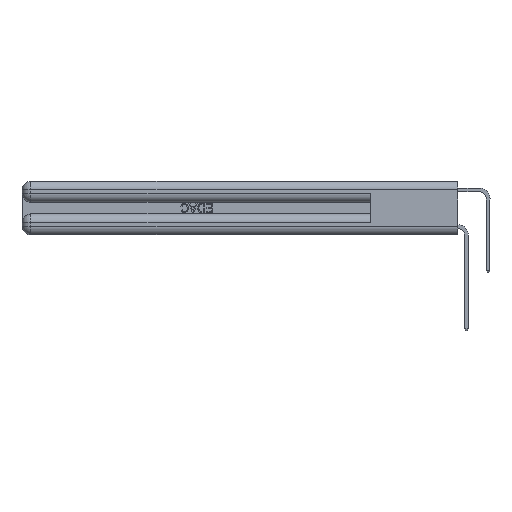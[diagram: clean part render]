
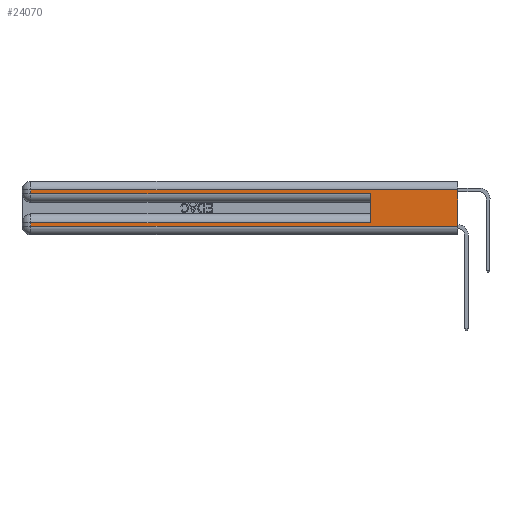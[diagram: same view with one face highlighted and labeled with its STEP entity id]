
A CAD part, left-side view. The second image highlights one B-rep face of the part: STEP entity #24070.
In plain terms, the highlighted planar face has unit normal (-1, 0, 0).
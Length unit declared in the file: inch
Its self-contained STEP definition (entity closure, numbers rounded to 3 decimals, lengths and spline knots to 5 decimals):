
#98 = EDGE_CURVE ( 'NONE', #16493, #9018, #6437, .T. ) ;
#126 = LINE ( 'NONE', #4403, #23424 ) ;
#523 = DIRECTION ( 'NONE',  ( 1., 0., 0. ) ) ;
#830 = VERTEX_POINT ( 'NONE', #20892 ) ;
#1413 = ORIENTED_EDGE ( 'NONE', *, *, #6226, .F. ) ;
#1420 = ORIENTED_EDGE ( 'NONE', *, *, #8567, .T. ) ;
#2170 = DIRECTION ( 'NONE',  ( 0., 0., -1. ) ) ;
#2882 = VERTEX_POINT ( 'NONE', #21152 ) ;
#3318 = CARTESIAN_POINT ( 'NONE',  ( 0., 0.6, 0.145 ) ) ;
#4073 = EDGE_CURVE ( 'NONE', #7418, #14097, #7111, .T. ) ;
#4253 = DIRECTION ( 'NONE',  ( 0., -1., 0. ) ) ;
#4347 = VECTOR ( 'NONE', #24216, 39.37008 ) ;
#4403 = CARTESIAN_POINT ( 'NONE',  ( 0., 0., 0.285 ) ) ;
#4581 = LINE ( 'NONE', #11133, #14206 ) ;
#4806 = CARTESIAN_POINT ( 'NONE',  ( 0., 0., 0.37 ) ) ;
#5591 = CARTESIAN_POINT ( 'NONE',  ( 0., 0., 0.31 ) ) ;
#5800 = CARTESIAN_POINT ( 'NONE',  ( 0., 2.94, 0.285 ) ) ;
#6103 = LINE ( 'NONE', #23733, #9230 ) ;
#6226 = EDGE_CURVE ( 'NONE', #2882, #830, #10009, .T. ) ;
#6437 = LINE ( 'NONE', #17681, #4347 ) ;
#6448 = EDGE_CURVE ( 'NONE', #18080, #24206, #4581, .T. ) ;
#6486 = EDGE_CURVE ( 'NONE', #2882, #16493, #17560, .T. ) ;
#6736 = CARTESIAN_POINT ( 'NONE',  ( 0., 0., 0.085 ) ) ;
#6940 = PLANE ( 'NONE',  #16130 ) ;
#7111 = LINE ( 'NONE', #9104, #25016 ) ;
#7418 = VERTEX_POINT ( 'NONE', #24120 ) ;
#8567 = EDGE_CURVE ( 'NONE', #9018, #14097, #6103, .T. ) ;
#8876 = CARTESIAN_POINT ( 'NONE',  ( 0., 2.94, 0.06 ) ) ;
#9018 = VERTEX_POINT ( 'NONE', #8876 ) ;
#9104 = CARTESIAN_POINT ( 'NONE',  ( 0., 0., 0.37 ) ) ;
#9214 = DIRECTION ( 'NONE',  ( 0., 0., -1. ) ) ;
#9230 = VECTOR ( 'NONE', #14782, 39.37008 ) ;
#9237 = ORIENTED_EDGE ( 'NONE', *, *, #98, .T. ) ;
#10009 = LINE ( 'NONE', #3318, #11490 ) ;
#10318 = VECTOR ( 'NONE', #18123, 39.37008 ) ;
#10510 = EDGE_CURVE ( 'NONE', #7418, #18080, #18402, .T. ) ;
#11133 = CARTESIAN_POINT ( 'NONE',  ( 0., 2.94, 0.37 ) ) ;
#11253 = EDGE_CURVE ( 'NONE', #24206, #830, #126, .T. ) ;
#11490 = VECTOR ( 'NONE', #27639, 39.37008 ) ;
#11905 = FACE_OUTER_BOUND ( 'NONE', #18092, .T. ) ;
#14062 = CARTESIAN_POINT ( 'NONE',  ( 0., 2.94, 0.085 ) ) ;
#14097 = VERTEX_POINT ( 'NONE', #20195 ) ;
#14142 = ORIENTED_EDGE ( 'NONE', *, *, #11253, .T. ) ;
#14206 = VECTOR ( 'NONE', #2170, 39.37008 ) ;
#14782 = DIRECTION ( 'NONE',  ( 0., -1., 0. ) ) ;
#15418 = DIRECTION ( 'NONE',  ( 0., 1., 0. ) ) ;
#16130 = AXIS2_PLACEMENT_3D ( 'NONE', #4806, #523, #9214 ) ;
#16493 = VERTEX_POINT ( 'NONE', #14062 ) ;
#17271 = CARTESIAN_POINT ( 'NONE',  ( 0., 2.94, 0.31 ) ) ;
#17560 = LINE ( 'NONE', #6736, #25509 ) ;
#17681 = CARTESIAN_POINT ( 'NONE',  ( 0., 2.94, 0.37 ) ) ;
#18080 = VERTEX_POINT ( 'NONE', #17271 ) ;
#18092 = EDGE_LOOP ( 'NONE', ( #25945, #22903, #26749, #14142, #1413, #25991, #9237, #1420 ) ) ;
#18123 = DIRECTION ( 'NONE',  ( 0., 1., 0. ) ) ;
#18402 = LINE ( 'NONE', #5591, #10318 ) ;
#20195 = CARTESIAN_POINT ( 'NONE',  ( 0., 0., 0.06 ) ) ;
#20892 = CARTESIAN_POINT ( 'NONE',  ( 0., 0.6, 0.285 ) ) ;
#21152 = CARTESIAN_POINT ( 'NONE',  ( 0., 0.6, 0.085 ) ) ;
#22903 = ORIENTED_EDGE ( 'NONE', *, *, #10510, .T. ) ;
#23424 = VECTOR ( 'NONE', #4253, 39.37008 ) ;
#23733 = CARTESIAN_POINT ( 'NONE',  ( 0., 0., 0.06 ) ) ;
#24070 = ADVANCED_FACE ( 'NONE', ( #11905 ), #6940, .F. ) ;
#24120 = CARTESIAN_POINT ( 'NONE',  ( 0., 0., 0.31 ) ) ;
#24206 = VERTEX_POINT ( 'NONE', #5800 ) ;
#24216 = DIRECTION ( 'NONE',  ( 0., 0., -1. ) ) ;
#24743 = DIRECTION ( 'NONE',  ( 0., 0., -1. ) ) ;
#25016 = VECTOR ( 'NONE', #24743, 39.37008 ) ;
#25509 = VECTOR ( 'NONE', #15418, 39.37008 ) ;
#25945 = ORIENTED_EDGE ( 'NONE', *, *, #4073, .F. ) ;
#25991 = ORIENTED_EDGE ( 'NONE', *, *, #6486, .T. ) ;
#26749 = ORIENTED_EDGE ( 'NONE', *, *, #6448, .T. ) ;
#27639 = DIRECTION ( 'NONE',  ( 0., 0., 1. ) ) ;
